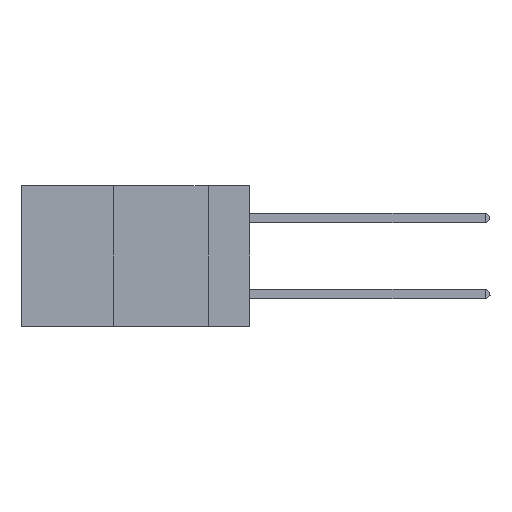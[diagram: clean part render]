
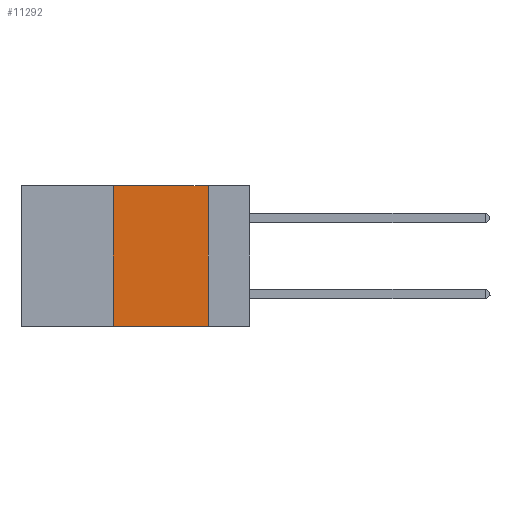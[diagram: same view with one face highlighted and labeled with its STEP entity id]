
A CAD part, left-side view. The second image highlights one B-rep face of the part: STEP entity #11292.
In plain terms, the highlighted planar face has unit normal (-1, 0, 0).
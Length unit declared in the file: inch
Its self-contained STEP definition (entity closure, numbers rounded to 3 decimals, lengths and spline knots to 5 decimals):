
#396 = EDGE_CURVE ( 'NONE', #17864, #19572, #8615, .T. ) ;
#1108 = ORIENTED_EDGE ( 'NONE', *, *, #14820, .F. ) ;
#2119 = CARTESIAN_POINT ( 'NONE',  ( 0., 0.36, 0. ) ) ;
#4270 = CARTESIAN_POINT ( 'NONE',  ( 0., 0.11, 0. ) ) ;
#5023 = VERTEX_POINT ( 'NONE', #4270 ) ;
#6290 = AXIS2_PLACEMENT_3D ( 'NONE', #14572, #21208, #10002 ) ;
#6924 = ORIENTED_EDGE ( 'NONE', *, *, #9337, .T. ) ;
#7319 = DIRECTION ( 'NONE',  ( 0., 0., -1. ) ) ;
#7462 = CARTESIAN_POINT ( 'NONE',  ( 0., 0.11, 0. ) ) ;
#7685 = EDGE_LOOP ( 'NONE', ( #15560, #1108, #20701, #6924 ) ) ;
#8031 = LINE ( 'NONE', #18189, #21198 ) ;
#8338 = CARTESIAN_POINT ( 'NONE',  ( 0., 0.36, 0. ) ) ;
#8615 = LINE ( 'NONE', #2119, #10959 ) ;
#9337 = EDGE_CURVE ( 'NONE', #17864, #17496, #11360, .T. ) ;
#9394 = VECTOR ( 'NONE', #7319, 39.37008 ) ;
#10002 = DIRECTION ( 'NONE',  ( 0., 0., -1. ) ) ;
#10616 = CARTESIAN_POINT ( 'NONE',  ( 0., 0.36, -0.37 ) ) ;
#10959 = VECTOR ( 'NONE', #12214, 39.37008 ) ;
#11292 = ADVANCED_FACE ( 'NONE', ( #20291 ), #15058, .F. ) ;
#11360 = LINE ( 'NONE', #15138, #15745 ) ;
#12214 = DIRECTION ( 'NONE',  ( 0., 0., 1. ) ) ;
#13086 = EDGE_CURVE ( 'NONE', #5023, #17496, #17122, .T. ) ;
#13563 = DIRECTION ( 'NONE',  ( 0., -1., 0. ) ) ;
#14243 = CARTESIAN_POINT ( 'NONE',  ( 0., 0.11, -0.37 ) ) ;
#14572 = CARTESIAN_POINT ( 'NONE',  ( 0., 0.6, 0. ) ) ;
#14820 = EDGE_CURVE ( 'NONE', #19572, #5023, #8031, .T. ) ;
#15058 = PLANE ( 'NONE',  #6290 ) ;
#15138 = CARTESIAN_POINT ( 'NONE',  ( 0., 0.6, -0.37 ) ) ;
#15560 = ORIENTED_EDGE ( 'NONE', *, *, #13086, .F. ) ;
#15745 = VECTOR ( 'NONE', #13563, 39.37008 ) ;
#17122 = LINE ( 'NONE', #7462, #9394 ) ;
#17496 = VERTEX_POINT ( 'NONE', #14243 ) ;
#17864 = VERTEX_POINT ( 'NONE', #10616 ) ;
#18189 = CARTESIAN_POINT ( 'NONE',  ( 0., 0.6, 0. ) ) ;
#19572 = VERTEX_POINT ( 'NONE', #8338 ) ;
#19848 = DIRECTION ( 'NONE',  ( 0., -1., 0. ) ) ;
#20291 = FACE_OUTER_BOUND ( 'NONE', #7685, .T. ) ;
#20701 = ORIENTED_EDGE ( 'NONE', *, *, #396, .F. ) ;
#21198 = VECTOR ( 'NONE', #19848, 39.37008 ) ;
#21208 = DIRECTION ( 'NONE',  ( 1., 0., 0. ) ) ;
